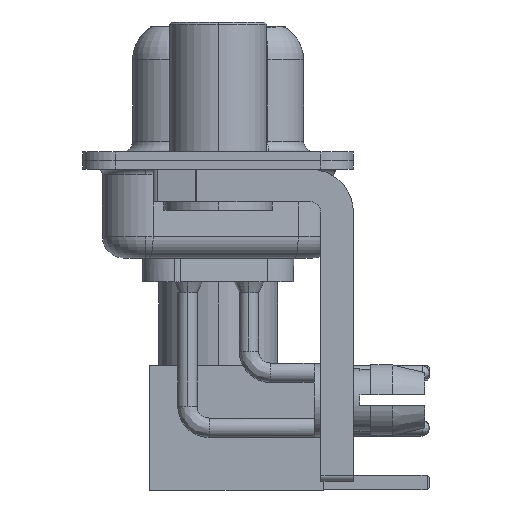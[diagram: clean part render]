
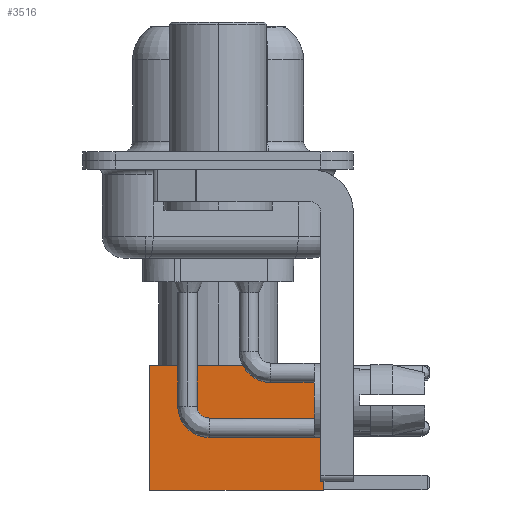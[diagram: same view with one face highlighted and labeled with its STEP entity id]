
A CAD part, left-side view. The second image highlights one B-rep face of the part: STEP entity #3516.
In plain terms, the highlighted face is planar.
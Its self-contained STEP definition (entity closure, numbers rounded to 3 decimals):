
#682 = CARTESIAN_POINT ( 'NONE',  ( 2.875, 2.875, 0. ) ) ;
#709 = CARTESIAN_POINT ( 'NONE',  ( 2.875, 2.875, 0. ) ) ;
#935 = LINE ( 'NONE', #12432, #24309 ) ;
#1130 = EDGE_CURVE ( 'NONE', #28988, #13960, #935, .T. ) ;
#1885 = ORIENTED_EDGE ( 'NONE', *, *, #1130, .F. ) ;
#3516 = ADVANCED_FACE ( 'NONE', ( #27907 ), #4780, .T. ) ;
#4780 = PLANE ( 'NONE',  #17194 ) ;
#5259 = DIRECTION ( 'NONE',  ( 0., 0., -1. ) ) ;
#5814 = EDGE_CURVE ( 'NONE', #28988, #10992, #23972, .T. ) ;
#6794 = EDGE_LOOP ( 'NONE', ( #7050, #27336, #29124, #1885 ) ) ;
#7050 = ORIENTED_EDGE ( 'NONE', *, *, #5814, .T. ) ;
#8831 = LINE ( 'NONE', #28951, #29820 ) ;
#10992 = VERTEX_POINT ( 'NONE', #21622 ) ;
#12033 = DIRECTION ( 'NONE',  ( 0., 0., 1. ) ) ;
#12275 = CARTESIAN_POINT ( 'NONE',  ( 0., 2.875, 0. ) ) ;
#12432 = CARTESIAN_POINT ( 'NONE',  ( 0., 2.875, 8. ) ) ;
#13960 = VERTEX_POINT ( 'NONE', #29760 ) ;
#15872 = VECTOR ( 'NONE', #24195, 1000. ) ;
#16654 = VERTEX_POINT ( 'NONE', #28034 ) ;
#16805 = DIRECTION ( 'NONE',  ( -1., 0., 0. ) ) ;
#17194 = AXIS2_PLACEMENT_3D ( 'NONE', #682, #25777, #12033 ) ;
#18035 = DIRECTION ( 'NONE',  ( 0., 0., -1. ) ) ;
#20727 = EDGE_CURVE ( 'NONE', #10992, #16654, #28603, .T. ) ;
#21622 = CARTESIAN_POINT ( 'NONE',  ( 2.875, 2.875, 0. ) ) ;
#22173 = CARTESIAN_POINT ( 'NONE',  ( 2.875, 2.875, 8. ) ) ;
#23972 = LINE ( 'NONE', #709, #25921 ) ;
#24195 = DIRECTION ( 'NONE',  ( -1., 0., 0. ) ) ;
#24309 = VECTOR ( 'NONE', #16805, 1000. ) ;
#25777 = DIRECTION ( 'NONE',  ( 0., 1., 0. ) ) ;
#25921 = VECTOR ( 'NONE', #5259, 1000. ) ;
#27336 = ORIENTED_EDGE ( 'NONE', *, *, #20727, .T. ) ;
#27364 = EDGE_CURVE ( 'NONE', #13960, #16654, #8831, .T. ) ;
#27907 = FACE_OUTER_BOUND ( 'NONE', #6794, .T. ) ;
#28034 = CARTESIAN_POINT ( 'NONE',  ( -2.875, 2.875, 0. ) ) ;
#28603 = LINE ( 'NONE', #12275, #15872 ) ;
#28951 = CARTESIAN_POINT ( 'NONE',  ( -2.875, 2.875, 0. ) ) ;
#28988 = VERTEX_POINT ( 'NONE', #22173 ) ;
#29124 = ORIENTED_EDGE ( 'NONE', *, *, #27364, .F. ) ;
#29760 = CARTESIAN_POINT ( 'NONE',  ( -2.875, 2.875, 8. ) ) ;
#29820 = VECTOR ( 'NONE', #18035, 1000. ) ;
